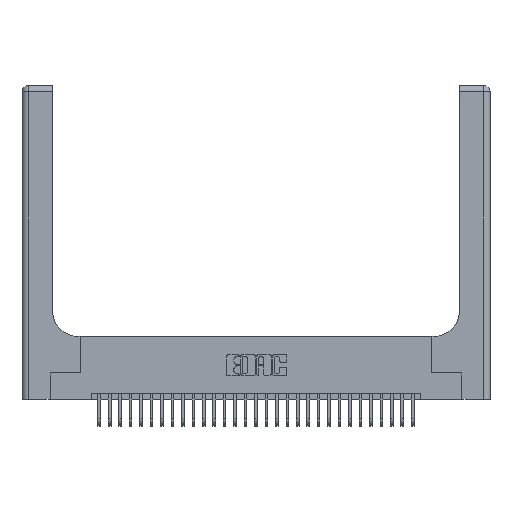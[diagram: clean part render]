
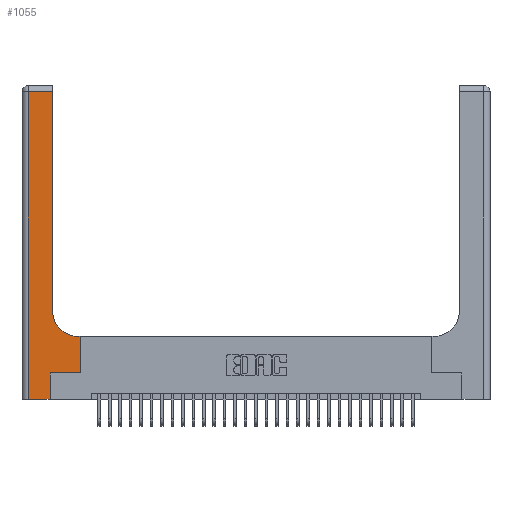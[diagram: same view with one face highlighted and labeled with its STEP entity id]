
A CAD part, top view. The second image highlights one B-rep face of the part: STEP entity #1055.
In plain terms, the highlighted planar face has unit normal (0, 0, 1).
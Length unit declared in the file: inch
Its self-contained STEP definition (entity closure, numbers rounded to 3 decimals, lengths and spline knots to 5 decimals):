
#620 = EDGE_CURVE ( 'NONE', #12821, #23164, #26575, .T. ) ;
#676 = CARTESIAN_POINT ( 'NONE',  ( 0.5585, 0.25, 0.37 ) ) ;
#1038 = CARTESIAN_POINT ( 'NONE',  ( 0.269, 0., 0.37 ) ) ;
#1055 = ADVANCED_FACE ( 'NONE', ( #24994 ), #13191, .F. ) ;
#1096 = EDGE_CURVE ( 'NONE', #4246, #8204, #2504, .T. ) ;
#1998 = CARTESIAN_POINT ( 'NONE',  ( 0.06, 2.94, 0.37 ) ) ;
#2073 = ORIENTED_EDGE ( 'NONE', *, *, #12912, .T. ) ;
#2188 = DIRECTION ( 'NONE',  ( 0., 0., -1. ) ) ;
#2504 = LINE ( 'NONE', #13291, #9592 ) ;
#2658 = CARTESIAN_POINT ( 'NONE',  ( 0., 0., 0.37 ) ) ;
#3035 = EDGE_CURVE ( 'NONE', #15587, #4246, #14964, .T. ) ;
#4117 = DIRECTION ( 'NONE',  ( 0., 1., 0. ) ) ;
#4168 = LINE ( 'NONE', #19381, #10451 ) ;
#4246 = VERTEX_POINT ( 'NONE', #1998 ) ;
#4619 = ORIENTED_EDGE ( 'NONE', *, *, #10300, .T. ) ;
#5965 = DIRECTION ( 'NONE',  ( -1., 0., 0. ) ) ;
#7575 = EDGE_CURVE ( 'NONE', #23164, #28635, #18561, .T. ) ;
#8204 = VERTEX_POINT ( 'NONE', #17504 ) ;
#9160 = EDGE_CURVE ( 'NONE', #22643, #22233, #15003, .T. ) ;
#9349 = ORIENTED_EDGE ( 'NONE', *, *, #620, .T. ) ;
#9460 = DIRECTION ( 'NONE',  ( 1., 0., 0. ) ) ;
#9592 = VECTOR ( 'NONE', #30583, 39.37008 ) ;
#10300 = EDGE_CURVE ( 'NONE', #8204, #22653, #25211, .T. ) ;
#10451 = VECTOR ( 'NONE', #27160, 39.37008 ) ;
#10747 = DIRECTION ( 'NONE',  ( 0., 0., -1. ) ) ;
#12821 = VERTEX_POINT ( 'NONE', #26303 ) ;
#12912 = EDGE_CURVE ( 'NONE', #28635, #22643, #4168, .T. ) ;
#13191 = PLANE ( 'NONE',  #15336 ) ;
#13291 = CARTESIAN_POINT ( 'NONE',  ( 0.06, 3., 0.37 ) ) ;
#13920 = ORIENTED_EDGE ( 'NONE', *, *, #3035, .T. ) ;
#14701 = DIRECTION ( 'NONE',  ( 0., 1., 0. ) ) ;
#14803 = CARTESIAN_POINT ( 'NONE',  ( 0.5585, 0.25, 0.37 ) ) ;
#14964 = LINE ( 'NONE', #15125, #20889 ) ;
#15003 = CIRCLE ( 'NONE', #18250, 0.25 ) ;
#15125 = CARTESIAN_POINT ( 'NONE',  ( 0., 2.94, 0.37 ) ) ;
#15336 = AXIS2_PLACEMENT_3D ( 'NONE', #20469, #10747, #30810 ) ;
#15568 = EDGE_LOOP ( 'NONE', ( #27327, #13920, #28065, #4619, #15623, #9349, #30257, #2073, #18435 ) ) ;
#15587 = VERTEX_POINT ( 'NONE', #18434 ) ;
#15623 = ORIENTED_EDGE ( 'NONE', *, *, #26168, .T. ) ;
#16606 = VECTOR ( 'NONE', #19060, 39.37008 ) ;
#17504 = CARTESIAN_POINT ( 'NONE',  ( 0.06, 0., 0.37 ) ) ;
#18179 = LINE ( 'NONE', #24234, #16606 ) ;
#18250 = AXIS2_PLACEMENT_3D ( 'NONE', #30628, #2188, #27966 ) ;
#18434 = CARTESIAN_POINT ( 'NONE',  ( 0.2915, 2.94, 0.37 ) ) ;
#18435 = ORIENTED_EDGE ( 'NONE', *, *, #9160, .T. ) ;
#18561 = LINE ( 'NONE', #14803, #24481 ) ;
#18703 = VECTOR ( 'NONE', #9460, 39.37008 ) ;
#19060 = DIRECTION ( 'NONE',  ( 0., 1., 0. ) ) ;
#19381 = CARTESIAN_POINT ( 'NONE',  ( 0.2915, 0.6, 0.37 ) ) ;
#20469 = CARTESIAN_POINT ( 'NONE',  ( 0., 3., 0.37 ) ) ;
#20889 = VECTOR ( 'NONE', #5965, 39.37008 ) ;
#22233 = VERTEX_POINT ( 'NONE', #29622 ) ;
#22643 = VERTEX_POINT ( 'NONE', #23541 ) ;
#22653 = VERTEX_POINT ( 'NONE', #1038 ) ;
#22961 = DIRECTION ( 'NONE',  ( 1., 0., 0. ) ) ;
#23164 = VERTEX_POINT ( 'NONE', #676 ) ;
#23269 = VECTOR ( 'NONE', #22961, 39.37008 ) ;
#23541 = CARTESIAN_POINT ( 'NONE',  ( 0.5415, 0.6, 0.37 ) ) ;
#23985 = LINE ( 'NONE', #29553, #31876 ) ;
#24234 = CARTESIAN_POINT ( 'NONE',  ( 0.269, 0., 0.37 ) ) ;
#24481 = VECTOR ( 'NONE', #14701, 39.37008 ) ;
#24994 = FACE_OUTER_BOUND ( 'NONE', #15568, .T. ) ;
#25211 = LINE ( 'NONE', #2658, #23269 ) ;
#25818 = CARTESIAN_POINT ( 'NONE',  ( 0.269, 0.25, 0.37 ) ) ;
#26168 = EDGE_CURVE ( 'NONE', #22653, #12821, #18179, .T. ) ;
#26303 = CARTESIAN_POINT ( 'NONE',  ( 0.269, 0.25, 0.37 ) ) ;
#26575 = LINE ( 'NONE', #25818, #18703 ) ;
#27160 = DIRECTION ( 'NONE',  ( -1., 0., 0. ) ) ;
#27327 = ORIENTED_EDGE ( 'NONE', *, *, #32661, .T. ) ;
#27966 = DIRECTION ( 'NONE',  ( 1., 0., 0. ) ) ;
#28065 = ORIENTED_EDGE ( 'NONE', *, *, #1096, .T. ) ;
#28635 = VERTEX_POINT ( 'NONE', #31157 ) ;
#29553 = CARTESIAN_POINT ( 'NONE',  ( 0.2915, 3., 0.37 ) ) ;
#29622 = CARTESIAN_POINT ( 'NONE',  ( 0.2915, 0.85, 0.37 ) ) ;
#30257 = ORIENTED_EDGE ( 'NONE', *, *, #7575, .T. ) ;
#30583 = DIRECTION ( 'NONE',  ( 0., -1., 0. ) ) ;
#30628 = CARTESIAN_POINT ( 'NONE',  ( 0.5415, 0.85, 0.37 ) ) ;
#30810 = DIRECTION ( 'NONE',  ( -1., 0., 0. ) ) ;
#31157 = CARTESIAN_POINT ( 'NONE',  ( 0.5585, 0.6, 0.37 ) ) ;
#31876 = VECTOR ( 'NONE', #4117, 39.37008 ) ;
#32661 = EDGE_CURVE ( 'NONE', #22233, #15587, #23985, .T. ) ;
